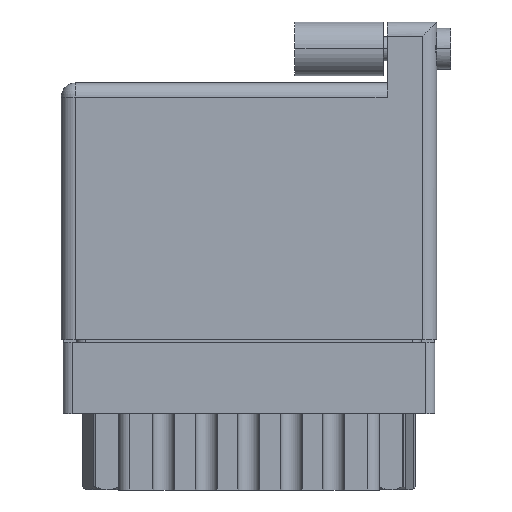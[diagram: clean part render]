
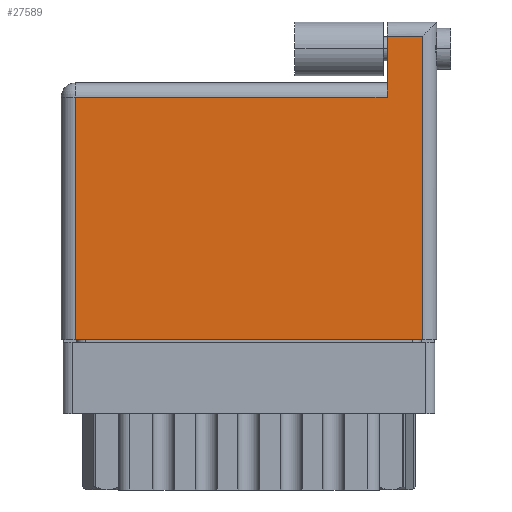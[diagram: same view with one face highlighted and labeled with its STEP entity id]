
A CAD part, front view. The second image highlights one B-rep face of the part: STEP entity #27589.
In plain terms, the highlighted face is planar.
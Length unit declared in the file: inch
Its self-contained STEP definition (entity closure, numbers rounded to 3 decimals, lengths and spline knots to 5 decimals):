
#516 = AXIS2_PLACEMENT_3D ( 'NONE', #35221, #5239, #26015 ) ;
#648 = ORIENTED_EDGE ( 'NONE', *, *, #23073, .T. ) ;
#1610 = ORIENTED_EDGE ( 'NONE', *, *, #29260, .T. ) ;
#2901 = CARTESIAN_POINT ( 'NONE',  ( 1.275, 1.07, 0. ) ) ;
#3707 = LINE ( 'NONE', #6020, #39014 ) ;
#4245 = CARTESIAN_POINT ( 'NONE',  ( 1.15, 1.12, 0. ) ) ;
#4347 = CARTESIAN_POINT ( 'NONE',  ( 0.05, 0., 0. ) ) ;
#4934 = CARTESIAN_POINT ( 'NONE',  ( 1.15, 1.07, 0. ) ) ;
#5239 = DIRECTION ( 'NONE',  ( 0., 0., -1. ) ) ;
#6020 = CARTESIAN_POINT ( 'NONE',  ( 0., 0.856, 0. ) ) ;
#7291 = VERTEX_POINT ( 'NONE', #27353 ) ;
#7694 = ORIENTED_EDGE ( 'NONE', *, *, #19950, .T. ) ;
#7803 = VERTEX_POINT ( 'NONE', #8800 ) ;
#8800 = CARTESIAN_POINT ( 'NONE',  ( 0.05, 0.856, 0. ) ) ;
#9097 = DIRECTION ( 'NONE',  ( -1., 0., 0. ) ) ;
#10111 = VECTOR ( 'NONE', #22566, 39.37008 ) ;
#10513 = VECTOR ( 'NONE', #25541, 39.37008 ) ;
#11351 = EDGE_CURVE ( 'NONE', #18291, #7291, #21260, .T. ) ;
#11858 = CARTESIAN_POINT ( 'NONE',  ( 1.275, 1.12, 0. ) ) ;
#12169 = CARTESIAN_POINT ( 'NONE',  ( 0.05, 0., 0. ) ) ;
#13231 = EDGE_CURVE ( 'NONE', #38092, #29672, #27441, .T. ) ;
#14801 = FACE_OUTER_BOUND ( 'NONE', #38496, .T. ) ;
#17255 = LINE ( 'NONE', #4347, #10111 ) ;
#17337 = PLANE ( 'NONE',  #516 ) ;
#17912 = VECTOR ( 'NONE', #21246, 39.37008 ) ;
#17945 = CARTESIAN_POINT ( 'NONE',  ( 0., 1.07, 0. ) ) ;
#18291 = VERTEX_POINT ( 'NONE', #12169 ) ;
#19950 = EDGE_CURVE ( 'NONE', #29672, #31786, #36715, .T. ) ;
#20126 = ORIENTED_EDGE ( 'NONE', *, *, #36951, .T. ) ;
#21246 = DIRECTION ( 'NONE',  ( -1., 0., 0. ) ) ;
#21260 = LINE ( 'NONE', #38615, #33216 ) ;
#22566 = DIRECTION ( 'NONE',  ( 0., -1., 0. ) ) ;
#23073 = EDGE_CURVE ( 'NONE', #7291, #38092, #37015, .T. ) ;
#23917 = CARTESIAN_POINT ( 'NONE',  ( 1.15, 0.856, 0. ) ) ;
#25541 = DIRECTION ( 'NONE',  ( 0., -1., 0. ) ) ;
#26015 = DIRECTION ( 'NONE',  ( -1., 0., 0. ) ) ;
#27030 = DIRECTION ( 'NONE',  ( 0., 1., 0. ) ) ;
#27353 = CARTESIAN_POINT ( 'NONE',  ( 1.275, 0., 0. ) ) ;
#27441 = LINE ( 'NONE', #17945, #17912 ) ;
#27589 = ADVANCED_FACE ( 'NONE', ( #14801 ), #17337, .F. ) ;
#27927 = ORIENTED_EDGE ( 'NONE', *, *, #11351, .T. ) ;
#29260 = EDGE_CURVE ( 'NONE', #31786, #7803, #3707, .T. ) ;
#29672 = VERTEX_POINT ( 'NONE', #4934 ) ;
#30311 = VECTOR ( 'NONE', #27030, 39.37008 ) ;
#30410 = ORIENTED_EDGE ( 'NONE', *, *, #13231, .T. ) ;
#31786 = VERTEX_POINT ( 'NONE', #23917 ) ;
#33009 = DIRECTION ( 'NONE',  ( 1., 0., 0. ) ) ;
#33216 = VECTOR ( 'NONE', #33009, 39.37008 ) ;
#35221 = CARTESIAN_POINT ( 'NONE',  ( 0., 0.906, 0. ) ) ;
#36715 = LINE ( 'NONE', #4245, #10513 ) ;
#36951 = EDGE_CURVE ( 'NONE', #7803, #18291, #17255, .T. ) ;
#37015 = LINE ( 'NONE', #11858, #30311 ) ;
#38092 = VERTEX_POINT ( 'NONE', #2901 ) ;
#38496 = EDGE_LOOP ( 'NONE', ( #27927, #648, #30410, #7694, #1610, #20126 ) ) ;
#38615 = CARTESIAN_POINT ( 'NONE',  ( 0., 0., 0. ) ) ;
#39014 = VECTOR ( 'NONE', #9097, 39.37008 ) ;
